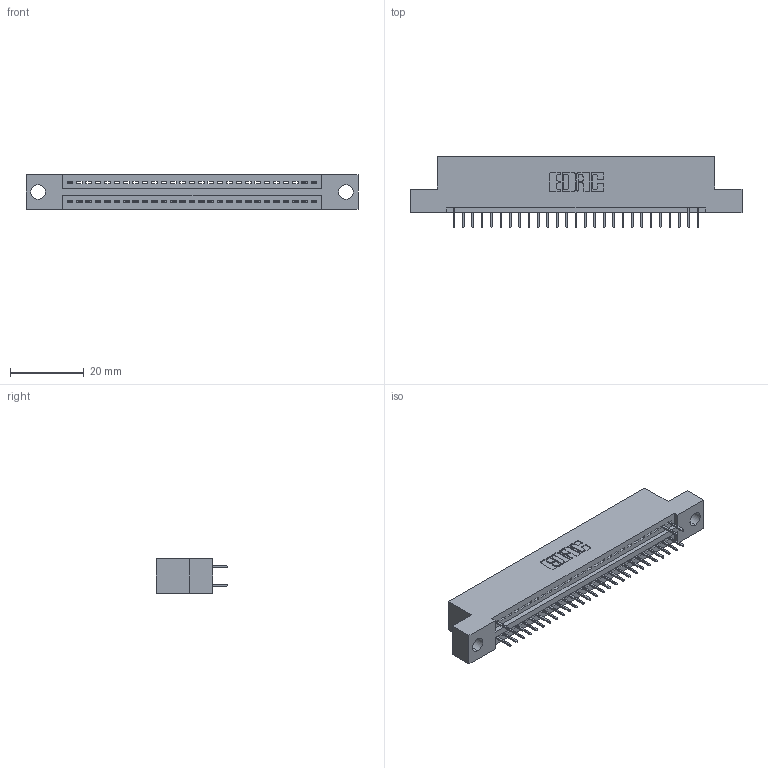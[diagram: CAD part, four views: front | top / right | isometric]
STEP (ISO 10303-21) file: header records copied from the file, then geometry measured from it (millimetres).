
FILE_DESCRIPTION (( 'STEP AP203' ), '1' );
FILE_NAME ('345-054-524-204.STEP', '2018-09-23T21:50:04', ( '' ), ( '' ), 'SwSTEP 2.0', 'SolidWorks 2016', '' );
FILE_SCHEMA (( 'CONFIG_CONTROL_DESIGN' ));
Length unit declared in the file: inch
Products named in the file (3): 345-292-001_345-293-124; 345-054-524-204; 345 Part_Flush Mounting Lugs - 0.156 Dia-TH
Assembly tree (31 placements, depth 2):
  345-054-524-204
    345 Part_Flush Mounting Lugs - 0.156 Dia-TH
    345-292-001_345-293-124  x30
Bounding box: 89.79 x 19.35 x 9.4 mm (x, y, z)
Volume: 8233.4 mm3; surface area: 10349.8 mm2
Topology: 31 solids, 31 shells, 1938 faces, 5579 edges, 3598 vertices
Faces by surface type: plane 1418, cylinder 520
Entity records: 22513 total; most frequent: CARTESIAN_POINT 3892, ORIENTED_EDGE 3850, DIRECTION 3425, EDGE_CURVE 1925, VECTOR 1689, LINE 1689, VERTEX_POINT 1278, AXIS2_PLACEMENT_3D 868
